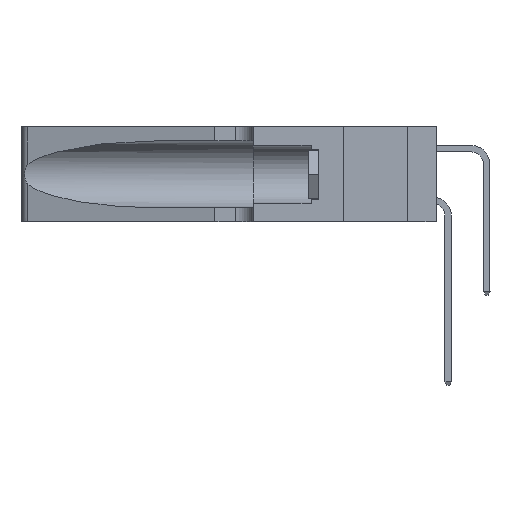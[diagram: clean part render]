
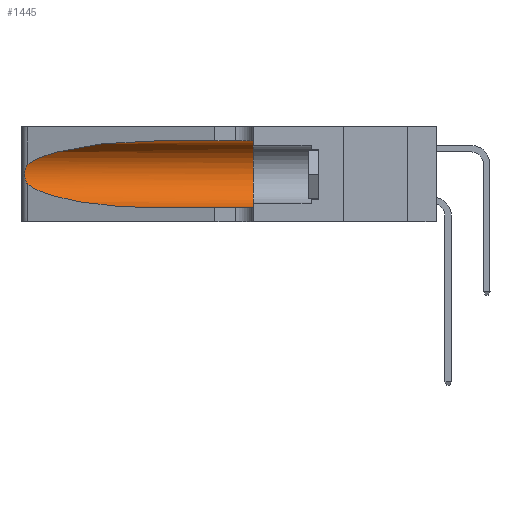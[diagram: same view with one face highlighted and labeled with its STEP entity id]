
A CAD part, left-side view. The second image highlights one B-rep face of the part: STEP entity #1445.
In plain terms, the highlighted cylindrical face has radius 3.308 mm (diameter 6.617 mm), a partial arc.
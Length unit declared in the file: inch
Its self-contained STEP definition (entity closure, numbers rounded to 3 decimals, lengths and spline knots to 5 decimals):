
#717 = VERTEX_POINT ( 'NONE', #11018 ) ;
#867 = CARTESIAN_POINT ( 'NONE',  ( 0.1305, 1.61858, 0.31525 ) ) ;
#1076 = ORIENTED_EDGE ( 'NONE', *, *, #2381, .F. ) ;
#1445 = ADVANCED_FACE ( 'NONE', ( #20894 ), #2879, .F. ) ;
#2381 = EDGE_CURVE ( 'NONE', #717, #3670, #16124, .T. ) ;
#2399 = B_SPLINE_CURVE_WITH_KNOTS ( 'NONE', 3,
 ( #18924, #30351, #23648, #14078, #16327, #11826, #4594, #21004, #11920, #28275, #4884, #9355, #23566, #13888 ),
 .UNSPECIFIED., .F., .F.,
 ( 4, 2, 2, 2, 2, 2, 4 ),
 ( 0., 0.00027, 0.00053, 0.00107, 0.0016, 0.00187, 0.00214 ),
 .UNSPECIFIED. ) ;
#2633 = DIRECTION ( 'NONE',  ( 0., 0., 1. ) ) ;
#2879 = CYLINDRICAL_SURFACE ( 'NONE', #24436, 0.13025 ) ;
#2973 = VERTEX_POINT ( 'NONE', #16986 ) ;
#2995 = CARTESIAN_POINT ( 'NONE',  ( 0.1305, 0.72297, 0.31525 ) ) ;
#3307 = CARTESIAN_POINT ( 'NONE',  ( 0.1305, 1.61858, 0.185 ) ) ;
#3670 = VERTEX_POINT ( 'NONE', #4660 ) ;
#3910 = ORIENTED_EDGE ( 'NONE', *, *, #12331, .T. ) ;
#4594 = CARTESIAN_POINT ( 'NONE',  ( 0.26075, 1.23896, 0.19203 ) ) ;
#4660 = CARTESIAN_POINT ( 'NONE',  ( 0.1305, 0.35, 0.31525 ) ) ;
#4884 = CARTESIAN_POINT ( 'NONE',  ( 0.25789, 1.23486, 0.15765 ) ) ;
#5060 =( BOUNDED_CURVE ( )  B_SPLINE_CURVE ( 3, ( #17409, #5700, #22102, #24456 ),
 .UNSPECIFIED., .F., .F. ) 
 B_SPLINE_CURVE_WITH_KNOTS ( ( 4, 4 ),
 ( 3.44316, 4.71239 ),
 .UNSPECIFIED. ) 
 CURVE ( )  GEOMETRIC_REPRESENTATION_ITEM ( )  RATIONAL_B_SPLINE_CURVE ( ( 1., 0.87, 0.87, 1. ) ) 
 REPRESENTATION_ITEM ( '' )  );
#5369 = CARTESIAN_POINT ( 'NONE',  ( 0.2373, 1.15595, 0.28018 ) ) ;
#5519 = VERTEX_POINT ( 'NONE', #6711 ) ;
#5700 = CARTESIAN_POINT ( 'NONE',  ( 0.2373, 1.15595, 0.08982 ) ) ;
#6257 = AXIS2_PLACEMENT_3D ( 'NONE', #26019, #12044, #2633 ) ;
#6711 = CARTESIAN_POINT ( 'NONE',  ( 0.1305, 0.72297, 0.05475 ) ) ;
#7270 = CARTESIAN_POINT ( 'NONE',  ( 0.18966, 0.96281, 0.31525 ) ) ;
#8177 = DIRECTION ( 'NONE',  ( 0., 0., -1. ) ) ;
#8261 = CARTESIAN_POINT ( 'NONE',  ( 0.25487, 1.22718, 0.14631 ) ) ;
#9355 = CARTESIAN_POINT ( 'NONE',  ( 0.25639, 1.23186, 0.15144 ) ) ;
#9514 = VECTOR ( 'NONE', #26856, 39.37008 ) ;
#10650 = ORIENTED_EDGE ( 'NONE', *, *, #27648, .F. ) ;
#11018 = CARTESIAN_POINT ( 'NONE',  ( 0.1305, 0.72297, 0.31525 ) ) ;
#11826 = CARTESIAN_POINT ( 'NONE',  ( 0.26018, 1.23835, 0.19895 ) ) ;
#11920 = CARTESIAN_POINT ( 'NONE',  ( 0.26017, 1.23833, 0.17102 ) ) ;
#12044 = DIRECTION ( 'NONE',  ( 0., 1., 0. ) ) ;
#12331 = EDGE_CURVE ( 'NONE', #717, #29939, #12432, .T. ) ;
#12432 =( BOUNDED_CURVE ( )  B_SPLINE_CURVE ( 3, ( #2995, #7270, #5369, #29066 ),
 .UNSPECIFIED., .F., .F. ) 
 B_SPLINE_CURVE_WITH_KNOTS ( ( 4, 4 ),
 ( 1.5708, 2.84003 ),
 .UNSPECIFIED. ) 
 CURVE ( )  GEOMETRIC_REPRESENTATION_ITEM ( )  RATIONAL_B_SPLINE_CURVE ( ( 1., 0.87, 0.87, 1. ) ) 
 REPRESENTATION_ITEM ( '' )  );
#13388 = EDGE_CURVE ( 'NONE', #25909, #5519, #5060, .T. ) ;
#13888 = CARTESIAN_POINT ( 'NONE',  ( 0.25487, 1.22718, 0.14631 ) ) ;
#14078 = CARTESIAN_POINT ( 'NONE',  ( 0.25787, 1.23484, 0.2124 ) ) ;
#14225 = EDGE_CURVE ( 'NONE', #5519, #2973, #19003, .T. ) ;
#16025 = EDGE_LOOP ( 'NONE', ( #3910, #21795, #29375, #23234, #10650, #1076 ) ) ;
#16124 = LINE ( 'NONE', #867, #27828 ) ;
#16327 = CARTESIAN_POINT ( 'NONE',  ( 0.25854, 1.2359, 0.20912 ) ) ;
#16986 = CARTESIAN_POINT ( 'NONE',  ( 0.1305, 0.35, 0.05475 ) ) ;
#17409 = CARTESIAN_POINT ( 'NONE',  ( 0.25487, 1.22718, 0.14631 ) ) ;
#18924 = CARTESIAN_POINT ( 'NONE',  ( 0.25487, 1.22718, 0.22369 ) ) ;
#18944 = CIRCLE ( 'NONE', #6257, 0.13025 ) ;
#19003 = LINE ( 'NONE', #22027, #9514 ) ;
#20018 = DIRECTION ( 'NONE',  ( 0., -1., 0. ) ) ;
#20095 = EDGE_CURVE ( 'NONE', #29939, #25909, #2399, .T. ) ;
#20894 = FACE_OUTER_BOUND ( 'NONE', #16025, .T. ) ;
#21004 = CARTESIAN_POINT ( 'NONE',  ( 0.26075, 1.23896, 0.178 ) ) ;
#21795 = ORIENTED_EDGE ( 'NONE', *, *, #20095, .T. ) ;
#22027 = CARTESIAN_POINT ( 'NONE',  ( 0.1305, 1.61858, 0.05475 ) ) ;
#22102 = CARTESIAN_POINT ( 'NONE',  ( 0.18966, 0.96281, 0.05475 ) ) ;
#23234 = ORIENTED_EDGE ( 'NONE', *, *, #14225, .T. ) ;
#23566 = CARTESIAN_POINT ( 'NONE',  ( 0.25555, 1.22993, 0.14849 ) ) ;
#23648 = CARTESIAN_POINT ( 'NONE',  ( 0.25639, 1.23184, 0.21858 ) ) ;
#24436 = AXIS2_PLACEMENT_3D ( 'NONE', #3307, #20018, #8177 ) ;
#24456 = CARTESIAN_POINT ( 'NONE',  ( 0.1305, 0.72297, 0.05475 ) ) ;
#24768 = CARTESIAN_POINT ( 'NONE',  ( 0.25487, 1.22718, 0.22369 ) ) ;
#25909 = VERTEX_POINT ( 'NONE', #8261 ) ;
#26019 = CARTESIAN_POINT ( 'NONE',  ( 0.1305, 0.35, 0.185 ) ) ;
#26636 = DIRECTION ( 'NONE',  ( 0., -1., 0. ) ) ;
#26856 = DIRECTION ( 'NONE',  ( 0., -1., 0. ) ) ;
#27648 = EDGE_CURVE ( 'NONE', #3670, #2973, #18944, .T. ) ;
#27828 = VECTOR ( 'NONE', #26636, 39.37008 ) ;
#28275 = CARTESIAN_POINT ( 'NONE',  ( 0.25856, 1.23593, 0.16098 ) ) ;
#29066 = CARTESIAN_POINT ( 'NONE',  ( 0.25487, 1.22718, 0.22369 ) ) ;
#29375 = ORIENTED_EDGE ( 'NONE', *, *, #13388, .T. ) ;
#29939 = VERTEX_POINT ( 'NONE', #24768 ) ;
#30351 = CARTESIAN_POINT ( 'NONE',  ( 0.25555, 1.22994, 0.2215 ) ) ;
